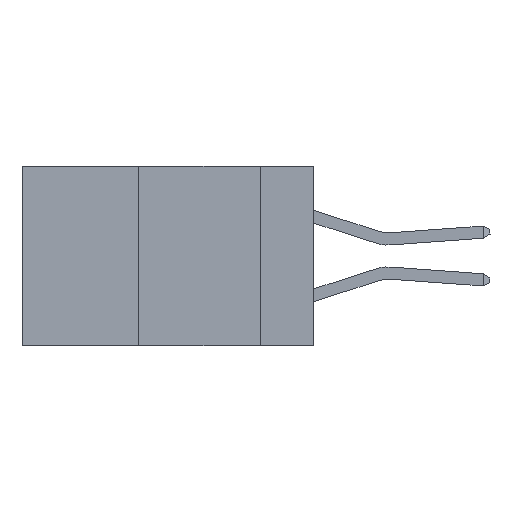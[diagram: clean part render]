
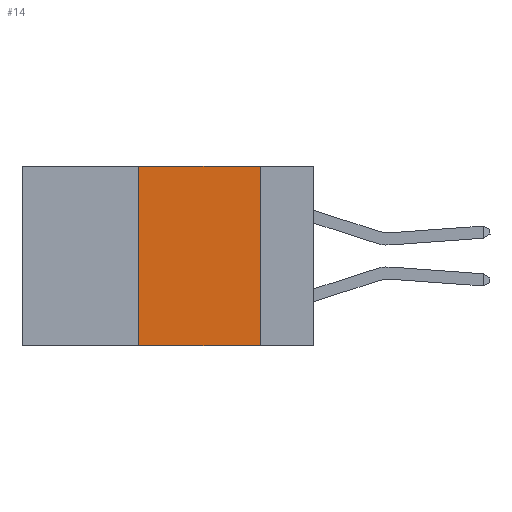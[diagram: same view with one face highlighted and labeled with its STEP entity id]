
A CAD part, left-side view. The second image highlights one B-rep face of the part: STEP entity #14.
In plain terms, the highlighted planar face has unit normal (-1, 0, 0).
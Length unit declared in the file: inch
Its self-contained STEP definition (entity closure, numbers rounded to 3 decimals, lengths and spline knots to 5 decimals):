
#14 = ADVANCED_FACE ( 'NONE', ( #25806 ), #3891, .F. ) ;
#2773 = EDGE_CURVE ( 'NONE', #7960, #17020, #11414, .T. ) ;
#3747 = AXIS2_PLACEMENT_3D ( 'NONE', #14743, #23735, #16304 ) ;
#3883 = DIRECTION ( 'NONE',  ( 0., -1., 0. ) ) ;
#3891 = PLANE ( 'NONE',  #3747 ) ;
#5931 = VERTEX_POINT ( 'NONE', #20539 ) ;
#7625 = EDGE_CURVE ( 'NONE', #10458, #7960, #10518, .T. ) ;
#7960 = VERTEX_POINT ( 'NONE', #11460 ) ;
#9254 = VECTOR ( 'NONE', #16317, 39.37008 ) ;
#9763 = VECTOR ( 'NONE', #25121, 39.37008 ) ;
#10458 = VERTEX_POINT ( 'NONE', #19127 ) ;
#10518 = LINE ( 'NONE', #24235, #9254 ) ;
#10757 = ORIENTED_EDGE ( 'NONE', *, *, #12484, .T. ) ;
#11414 = LINE ( 'NONE', #25779, #16052 ) ;
#11460 = CARTESIAN_POINT ( 'NONE',  ( 0., 0.36, 0. ) ) ;
#12484 = EDGE_CURVE ( 'NONE', #10458, #5931, #12781, .T. ) ;
#12781 = LINE ( 'NONE', #13473, #22728 ) ;
#13126 = ORIENTED_EDGE ( 'NONE', *, *, #2773, .F. ) ;
#13473 = CARTESIAN_POINT ( 'NONE',  ( 0., 0.6, -0.37 ) ) ;
#14743 = CARTESIAN_POINT ( 'NONE',  ( 0., 0.6, 0. ) ) ;
#16052 = VECTOR ( 'NONE', #3883, 39.37008 ) ;
#16304 = DIRECTION ( 'NONE',  ( 0., 0., -1. ) ) ;
#16317 = DIRECTION ( 'NONE',  ( 0., 0., 1. ) ) ;
#17014 = ORIENTED_EDGE ( 'NONE', *, *, #7625, .F. ) ;
#17020 = VERTEX_POINT ( 'NONE', #22865 ) ;
#17127 = EDGE_CURVE ( 'NONE', #17020, #5931, #25620, .T. ) ;
#19127 = CARTESIAN_POINT ( 'NONE',  ( 0., 0.36, -0.37 ) ) ;
#19196 = ORIENTED_EDGE ( 'NONE', *, *, #17127, .F. ) ;
#20539 = CARTESIAN_POINT ( 'NONE',  ( 0., 0.11, -0.37 ) ) ;
#22728 = VECTOR ( 'NONE', #25455, 39.37008 ) ;
#22865 = CARTESIAN_POINT ( 'NONE',  ( 0., 0.11, 0. ) ) ;
#23132 = CARTESIAN_POINT ( 'NONE',  ( 0., 0.11, 0. ) ) ;
#23602 = EDGE_LOOP ( 'NONE', ( #19196, #13126, #17014, #10757 ) ) ;
#23735 = DIRECTION ( 'NONE',  ( 1., 0., 0. ) ) ;
#24235 = CARTESIAN_POINT ( 'NONE',  ( 0., 0.36, 0. ) ) ;
#25121 = DIRECTION ( 'NONE',  ( 0., 0., -1. ) ) ;
#25455 = DIRECTION ( 'NONE',  ( 0., -1., 0. ) ) ;
#25620 = LINE ( 'NONE', #23132, #9763 ) ;
#25779 = CARTESIAN_POINT ( 'NONE',  ( 0., 0.6, 0. ) ) ;
#25806 = FACE_OUTER_BOUND ( 'NONE', #23602, .T. ) ;
